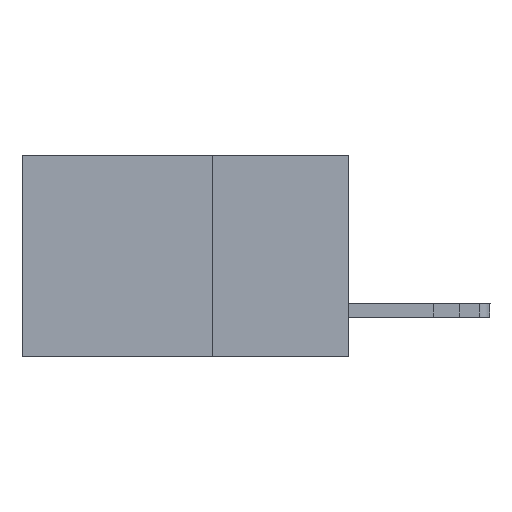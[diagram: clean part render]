
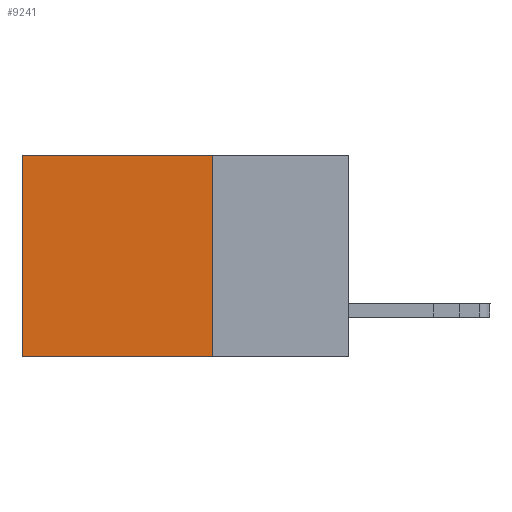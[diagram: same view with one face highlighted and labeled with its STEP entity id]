
A CAD part, left-side view. The second image highlights one B-rep face of the part: STEP entity #9241.
In plain terms, the highlighted planar face has unit normal (-1, 0, 0).
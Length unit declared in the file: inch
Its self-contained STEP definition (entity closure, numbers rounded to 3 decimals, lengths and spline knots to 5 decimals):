
#459 = CARTESIAN_POINT ( 'NONE',  ( 0.2615, 0.25, -0.37 ) ) ;
#486 = DIRECTION ( 'NONE',  ( 0., 0., -1. ) ) ;
#781 = DIRECTION ( 'NONE',  ( 0., 0., -1. ) ) ;
#1300 = LINE ( 'NONE', #16173, #8151 ) ;
#1791 = ORIENTED_EDGE ( 'NONE', *, *, #12357, .F. ) ;
#3030 = LINE ( 'NONE', #6990, #11296 ) ;
#4428 = ORIENTED_EDGE ( 'NONE', *, *, #12290, .T. ) ;
#6093 = VERTEX_POINT ( 'NONE', #6408 ) ;
#6408 = CARTESIAN_POINT ( 'NONE',  ( 0.2615, 0.25, 0. ) ) ;
#6829 = ORIENTED_EDGE ( 'NONE', *, *, #7792, .T. ) ;
#6990 = CARTESIAN_POINT ( 'NONE',  ( 0.2615, 0.25, -0.37 ) ) ;
#7792 = EDGE_CURVE ( 'NONE', #7895, #9946, #9036, .T. ) ;
#7895 = VERTEX_POINT ( 'NONE', #10063 ) ;
#8151 = VECTOR ( 'NONE', #13033, 39.37008 ) ;
#8360 = LINE ( 'NONE', #459, #12503 ) ;
#9036 = LINE ( 'NONE', #19035, #12694 ) ;
#9241 = ADVANCED_FACE ( 'NONE', ( #18337 ), #19317, .F. ) ;
#9826 = DIRECTION ( 'NONE',  ( 0., 1., 0. ) ) ;
#9946 = VERTEX_POINT ( 'NONE', #11686 ) ;
#10019 = AXIS2_PLACEMENT_3D ( 'NONE', #17817, #10150, #781 ) ;
#10063 = CARTESIAN_POINT ( 'NONE',  ( 0.2615, 0.6, 0. ) ) ;
#10150 = DIRECTION ( 'NONE',  ( 1., 0., 0. ) ) ;
#11296 = VECTOR ( 'NONE', #11728, 39.37008 ) ;
#11686 = CARTESIAN_POINT ( 'NONE',  ( 0.2615, 0.6, -0.37 ) ) ;
#11728 = DIRECTION ( 'NONE',  ( 0., 0., -1. ) ) ;
#12290 = EDGE_CURVE ( 'NONE', #6093, #7895, #1300, .T. ) ;
#12357 = EDGE_CURVE ( 'NONE', #6093, #16260, #3030, .T. ) ;
#12503 = VECTOR ( 'NONE', #9826, 39.37008 ) ;
#12694 = VECTOR ( 'NONE', #486, 39.37008 ) ;
#13033 = DIRECTION ( 'NONE',  ( 0., 1., 0. ) ) ;
#13833 = CARTESIAN_POINT ( 'NONE',  ( 0.2615, 0.25, -0.37 ) ) ;
#16173 = CARTESIAN_POINT ( 'NONE',  ( 0.2615, 0.25, 0. ) ) ;
#16260 = VERTEX_POINT ( 'NONE', #13833 ) ;
#17171 = EDGE_CURVE ( 'NONE', #16260, #9946, #8360, .T. ) ;
#17817 = CARTESIAN_POINT ( 'NONE',  ( 0.2615, 0.25, -0.37 ) ) ;
#18109 = ORIENTED_EDGE ( 'NONE', *, *, #17171, .F. ) ;
#18337 = FACE_OUTER_BOUND ( 'NONE', #18973, .T. ) ;
#18973 = EDGE_LOOP ( 'NONE', ( #6829, #18109, #1791, #4428 ) ) ;
#19035 = CARTESIAN_POINT ( 'NONE',  ( 0.2615, 0.6, -0.37 ) ) ;
#19317 = PLANE ( 'NONE',  #10019 ) ;
